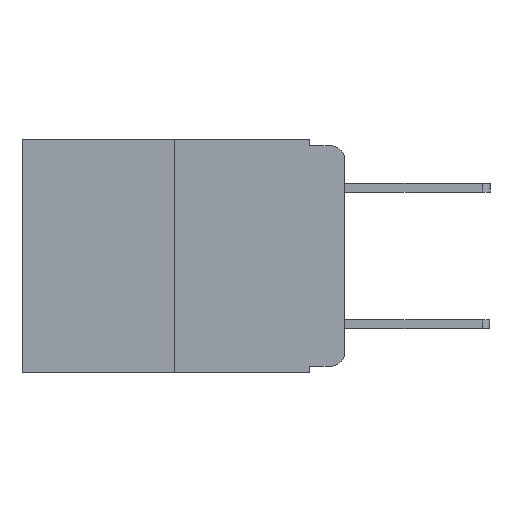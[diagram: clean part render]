
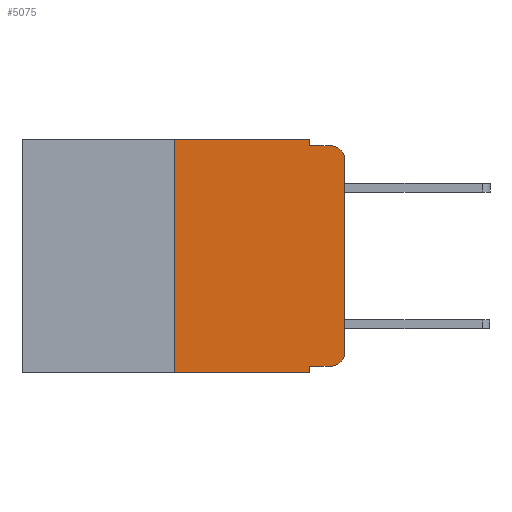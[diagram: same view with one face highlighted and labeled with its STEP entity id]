
A CAD part, left-side view. The second image highlights one B-rep face of the part: STEP entity #5075.
In plain terms, the highlighted planar face has unit normal (-1, 0, 0).
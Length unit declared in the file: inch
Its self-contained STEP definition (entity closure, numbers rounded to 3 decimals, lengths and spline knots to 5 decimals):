
#74 = CARTESIAN_POINT ( 'NONE',  ( 0., 0.473, -0.343 ) ) ;
#124 = AXIS2_PLACEMENT_3D ( 'NONE', #6233, #1227, #7019 ) ;
#182 = DIRECTION ( 'NONE',  ( 0., -1., 0. ) ) ;
#391 = LINE ( 'NONE', #74, #8885 ) ;
#473 = CARTESIAN_POINT ( 'NONE',  ( 0., 0.02, -0.01 ) ) ;
#797 = VECTOR ( 'NONE', #9806, 39.37008 ) ;
#900 = VECTOR ( 'NONE', #7872, 39.37008 ) ;
#966 = VERTEX_POINT ( 'NONE', #6792 ) ;
#1036 = EDGE_CURVE ( 'NONE', #2696, #3251, #7735, .T. ) ;
#1115 = LINE ( 'NONE', #6820, #797 ) ;
#1132 = ORIENTED_EDGE ( 'NONE', *, *, #10315, .T. ) ;
#1217 = EDGE_CURVE ( 'NONE', #6187, #966, #391, .T. ) ;
#1227 = DIRECTION ( 'NONE',  ( -1., 0., 0. ) ) ;
#1477 = ORIENTED_EDGE ( 'NONE', *, *, #9481, .F. ) ;
#1491 = ORIENTED_EDGE ( 'NONE', *, *, #1217, .T. ) ;
#1529 = ORIENTED_EDGE ( 'NONE', *, *, #4190, .F. ) ;
#1743 = VERTEX_POINT ( 'NONE', #8639 ) ;
#1858 = ORIENTED_EDGE ( 'NONE', *, *, #3646, .T. ) ;
#1986 = VERTEX_POINT ( 'NONE', #4122 ) ;
#1999 = VECTOR ( 'NONE', #5041, 39.37008 ) ;
#2028 = CIRCLE ( 'NONE', #5657, 0.02 ) ;
#2279 = CARTESIAN_POINT ( 'NONE',  ( 0., 0.473, 0. ) ) ;
#2413 = VERTEX_POINT ( 'NONE', #473 ) ;
#2576 = CARTESIAN_POINT ( 'NONE',  ( 0., 0.02, -0.03 ) ) ;
#2626 = AXIS2_PLACEMENT_3D ( 'NONE', #2279, #7859, #3160 ) ;
#2696 = VERTEX_POINT ( 'NONE', #6981 ) ;
#2998 = CARTESIAN_POINT ( 'NONE',  ( 0., 0., -0.313 ) ) ;
#3160 = DIRECTION ( 'NONE',  ( 0., 0., -1. ) ) ;
#3251 = VERTEX_POINT ( 'NONE', #3268 ) ;
#3257 = LINE ( 'NONE', #4268, #7213 ) ;
#3268 = CARTESIAN_POINT ( 'NONE',  ( 0., 0.051, 0. ) ) ;
#3345 = ORIENTED_EDGE ( 'NONE', *, *, #1036, .F. ) ;
#3453 = DIRECTION ( 'NONE',  ( 0., 0., -1. ) ) ;
#3646 = EDGE_CURVE ( 'NONE', #5665, #1743, #7509, .T. ) ;
#3690 = CARTESIAN_POINT ( 'NONE',  ( 0., 0.051, -0.333 ) ) ;
#3696 = DIRECTION ( 'NONE',  ( 0., -1., 0. ) ) ;
#3852 = ORIENTED_EDGE ( 'NONE', *, *, #8011, .F. ) ;
#4122 = CARTESIAN_POINT ( 'NONE',  ( 0., 0.051, -0.01 ) ) ;
#4190 = EDGE_CURVE ( 'NONE', #1986, #2413, #8999, .T. ) ;
#4207 = CARTESIAN_POINT ( 'NONE',  ( 0., 0.051, 0. ) ) ;
#4268 = CARTESIAN_POINT ( 'NONE',  ( 0., 0.25, 0. ) ) ;
#4306 = CARTESIAN_POINT ( 'NONE',  ( 0., 0.051, -0.01 ) ) ;
#4670 = CIRCLE ( 'NONE', #124, 0.02 ) ;
#5041 = DIRECTION ( 'NONE',  ( 0., 0., -1. ) ) ;
#5075 = ADVANCED_FACE ( 'NONE', ( #9320 ), #9055, .F. ) ;
#5101 = DIRECTION ( 'NONE',  ( 0., 0., 1. ) ) ;
#5319 = CARTESIAN_POINT ( 'NONE',  ( 0., 0.25, -0.343 ) ) ;
#5324 = VERTEX_POINT ( 'NONE', #2998 ) ;
#5475 = VECTOR ( 'NONE', #9408, 39.37008 ) ;
#5657 = AXIS2_PLACEMENT_3D ( 'NONE', #2576, #8117, #3453 ) ;
#5665 = VERTEX_POINT ( 'NONE', #3690 ) ;
#5880 = VECTOR ( 'NONE', #9473, 39.37008 ) ;
#5947 = VECTOR ( 'NONE', #3696, 39.37008 ) ;
#6123 = LINE ( 'NONE', #8743, #5880 ) ;
#6187 = VERTEX_POINT ( 'NONE', #5319 ) ;
#6233 = CARTESIAN_POINT ( 'NONE',  ( 0., 0.02, -0.313 ) ) ;
#6766 = VERTEX_POINT ( 'NONE', #7743 ) ;
#6792 = CARTESIAN_POINT ( 'NONE',  ( 0., 0.051, -0.343 ) ) ;
#6820 = CARTESIAN_POINT ( 'NONE',  ( 0., 0., 0. ) ) ;
#6981 = CARTESIAN_POINT ( 'NONE',  ( 0., 0.25, 0. ) ) ;
#7019 = DIRECTION ( 'NONE',  ( 0., 0., -1. ) ) ;
#7213 = VECTOR ( 'NONE', #5101, 39.37008 ) ;
#7421 = ORIENTED_EDGE ( 'NONE', *, *, #7515, .T. ) ;
#7509 = LINE ( 'NONE', #7973, #900 ) ;
#7515 = EDGE_CURVE ( 'NONE', #6766, #2413, #2028, .T. ) ;
#7735 = LINE ( 'NONE', #9201, #5947 ) ;
#7743 = CARTESIAN_POINT ( 'NONE',  ( 0., 0., -0.03 ) ) ;
#7859 = DIRECTION ( 'NONE',  ( 1., 0., 0. ) ) ;
#7872 = DIRECTION ( 'NONE',  ( 0., -1., 0. ) ) ;
#7973 = CARTESIAN_POINT ( 'NONE',  ( 0., 0.051, -0.333 ) ) ;
#8009 = ORIENTED_EDGE ( 'NONE', *, *, #10518, .F. ) ;
#8011 = EDGE_CURVE ( 'NONE', #3251, #1986, #6123, .T. ) ;
#8111 = ORIENTED_EDGE ( 'NONE', *, *, #10238, .T. ) ;
#8117 = DIRECTION ( 'NONE',  ( -1., 0., 0. ) ) ;
#8354 = LINE ( 'NONE', #4207, #1999 ) ;
#8639 = CARTESIAN_POINT ( 'NONE',  ( 0., 0.02, -0.333 ) ) ;
#8721 = EDGE_LOOP ( 'NONE', ( #8111, #7421, #1529, #3852, #3345, #1477, #1491, #8009, #1858, #1132 ) ) ;
#8743 = CARTESIAN_POINT ( 'NONE',  ( 0., 0.051, 0. ) ) ;
#8885 = VECTOR ( 'NONE', #182, 39.37008 ) ;
#8999 = LINE ( 'NONE', #4306, #5475 ) ;
#9055 = PLANE ( 'NONE',  #2626 ) ;
#9201 = CARTESIAN_POINT ( 'NONE',  ( 0., 0.473, 0. ) ) ;
#9320 = FACE_OUTER_BOUND ( 'NONE', #8721, .T. ) ;
#9408 = DIRECTION ( 'NONE',  ( 0., -1., 0. ) ) ;
#9473 = DIRECTION ( 'NONE',  ( 0., 0., -1. ) ) ;
#9481 = EDGE_CURVE ( 'NONE', #6187, #2696, #3257, .T. ) ;
#9806 = DIRECTION ( 'NONE',  ( 0., 0., 1. ) ) ;
#10238 = EDGE_CURVE ( 'NONE', #5324, #6766, #1115, .T. ) ;
#10315 = EDGE_CURVE ( 'NONE', #1743, #5324, #4670, .T. ) ;
#10518 = EDGE_CURVE ( 'NONE', #5665, #966, #8354, .T. ) ;
